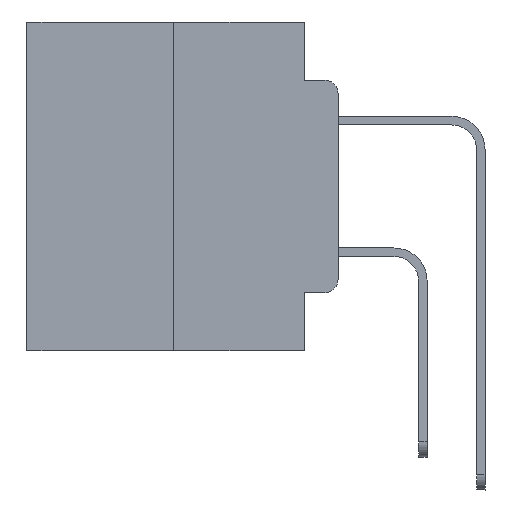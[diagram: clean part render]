
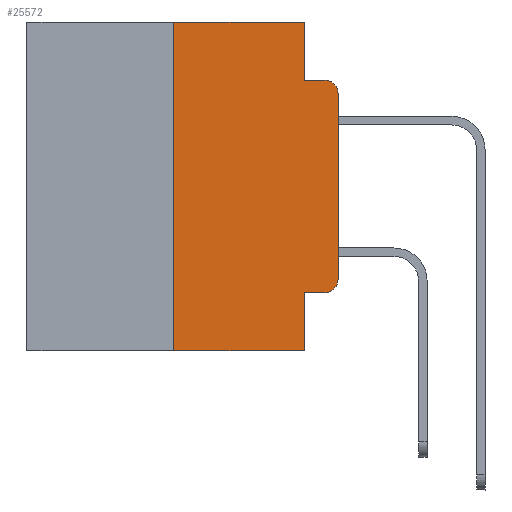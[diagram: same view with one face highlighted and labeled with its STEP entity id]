
A CAD part, left-side view. The second image highlights one B-rep face of the part: STEP entity #25572.
In plain terms, the highlighted planar face has unit normal (-1, 0, 0).
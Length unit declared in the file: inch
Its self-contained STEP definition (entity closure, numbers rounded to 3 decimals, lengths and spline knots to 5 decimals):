
#29 = DIRECTION ( 'NONE',  ( 0., -1., 0. ) ) ;
#83 = DIRECTION ( 'NONE',  ( 0., -1., 0. ) ) ;
#188 = EDGE_CURVE ( 'NONE', #13512, #18082, #9195, .T. ) ;
#240 = CARTESIAN_POINT ( 'NONE',  ( 0., 0.051, -0.0885 ) ) ;
#314 = CARTESIAN_POINT ( 'NONE',  ( 0., 0.02, -0.0885 ) ) ;
#466 = CARTESIAN_POINT ( 'NONE',  ( 0., 0.051, 0. ) ) ;
#577 = CARTESIAN_POINT ( 'NONE',  ( 0., 0.051, -0.0885 ) ) ;
#767 = CIRCLE ( 'NONE', #22059, 0.02 ) ;
#892 = CARTESIAN_POINT ( 'NONE',  ( 0., 0., 0. ) ) ;
#1604 = AXIS2_PLACEMENT_3D ( 'NONE', #3013, #21350, #19277 ) ;
#2238 = EDGE_CURVE ( 'NONE', #17097, #25896, #7556, .T. ) ;
#2462 = CARTESIAN_POINT ( 'NONE',  ( 0., 0.051, -0.4115 ) ) ;
#2566 = CARTESIAN_POINT ( 'NONE',  ( 0., 0.25, -0.5 ) ) ;
#3013 = CARTESIAN_POINT ( 'NONE',  ( 0., 0.02, -0.3915 ) ) ;
#3143 = CARTESIAN_POINT ( 'NONE',  ( 0., 0.25, 0. ) ) ;
#3380 = ORIENTED_EDGE ( 'NONE', *, *, #3652, .F. ) ;
#3582 = CARTESIAN_POINT ( 'NONE',  ( 0., 0.473, 0. ) ) ;
#3652 = EDGE_CURVE ( 'NONE', #5473, #27436, #4929, .T. ) ;
#3845 = CARTESIAN_POINT ( 'NONE',  ( 0., 0., -0.1085 ) ) ;
#3953 = VECTOR ( 'NONE', #27276, 39.37008 ) ;
#4034 = FACE_OUTER_BOUND ( 'NONE', #17146, .T. ) ;
#4355 = LINE ( 'NONE', #24919, #13659 ) ;
#4866 = CARTESIAN_POINT ( 'NONE',  ( 0., 0.25, 0. ) ) ;
#4929 = LINE ( 'NONE', #3143, #11040 ) ;
#5051 = ORIENTED_EDGE ( 'NONE', *, *, #12981, .T. ) ;
#5473 = VERTEX_POINT ( 'NONE', #2566 ) ;
#6499 = VERTEX_POINT ( 'NONE', #314 ) ;
#7221 = ORIENTED_EDGE ( 'NONE', *, *, #29108, .T. ) ;
#7556 = LINE ( 'NONE', #466, #18891 ) ;
#7664 = ORIENTED_EDGE ( 'NONE', *, *, #13264, .F. ) ;
#7984 = ORIENTED_EDGE ( 'NONE', *, *, #2238, .F. ) ;
#8680 = DIRECTION ( 'NONE',  ( -1., 0., 0. ) ) ;
#9007 = EDGE_CURVE ( 'NONE', #5473, #18082, #4355, .T. ) ;
#9189 = VERTEX_POINT ( 'NONE', #19699 ) ;
#9195 = LINE ( 'NONE', #18223, #3953 ) ;
#9214 = DIRECTION ( 'NONE',  ( 0., 0., 1. ) ) ;
#9650 = VERTEX_POINT ( 'NONE', #3845 ) ;
#10762 = CARTESIAN_POINT ( 'NONE',  ( 0., 0.02, -0.1085 ) ) ;
#10862 = DIRECTION ( 'NONE',  ( 0., -1., 0. ) ) ;
#11040 = VECTOR ( 'NONE', #9214, 39.37008 ) ;
#11886 = EDGE_CURVE ( 'NONE', #13512, #12898, #16207, .T. ) ;
#12185 = ORIENTED_EDGE ( 'NONE', *, *, #20729, .F. ) ;
#12315 = ORIENTED_EDGE ( 'NONE', *, *, #12469, .T. ) ;
#12469 = EDGE_CURVE ( 'NONE', #12898, #9189, #27140, .T. ) ;
#12898 = VERTEX_POINT ( 'NONE', #19241 ) ;
#12981 = EDGE_CURVE ( 'NONE', #9189, #9650, #23250, .T. ) ;
#13042 = PLANE ( 'NONE',  #25660 ) ;
#13235 = LINE ( 'NONE', #17503, #15631 ) ;
#13264 = EDGE_CURVE ( 'NONE', #25896, #6499, #22744, .T. ) ;
#13512 = VERTEX_POINT ( 'NONE', #26000 ) ;
#13659 = VECTOR ( 'NONE', #29, 39.37008 ) ;
#14627 = ORIENTED_EDGE ( 'NONE', *, *, #11886, .T. ) ;
#15631 = VECTOR ( 'NONE', #10862, 39.37008 ) ;
#15754 = CARTESIAN_POINT ( 'NONE',  ( 0., 0.051, -0.5 ) ) ;
#16207 = LINE ( 'NONE', #2462, #19534 ) ;
#17012 = DIRECTION ( 'NONE',  ( 0., 0., -1. ) ) ;
#17097 = VERTEX_POINT ( 'NONE', #19285 ) ;
#17146 = EDGE_LOOP ( 'NONE', ( #5051, #7221, #7664, #7984, #12185, #3380, #25011, #22921, #14627, #12315 ) ) ;
#17503 = CARTESIAN_POINT ( 'NONE',  ( 0., 0.473, 0. ) ) ;
#18082 = VERTEX_POINT ( 'NONE', #15754 ) ;
#18223 = CARTESIAN_POINT ( 'NONE',  ( 0., 0.051, 0. ) ) ;
#18236 = DIRECTION ( 'NONE',  ( 0., 0., -1. ) ) ;
#18891 = VECTOR ( 'NONE', #18236, 39.37008 ) ;
#19241 = CARTESIAN_POINT ( 'NONE',  ( 0., 0.02, -0.4115 ) ) ;
#19277 = DIRECTION ( 'NONE',  ( 0., 0., -1. ) ) ;
#19285 = CARTESIAN_POINT ( 'NONE',  ( 0., 0.051, 0. ) ) ;
#19534 = VECTOR ( 'NONE', #83, 39.37008 ) ;
#19699 = CARTESIAN_POINT ( 'NONE',  ( 0., 0., -0.3915 ) ) ;
#20729 = EDGE_CURVE ( 'NONE', #27436, #17097, #13235, .T. ) ;
#21350 = DIRECTION ( 'NONE',  ( -1., 0., 0. ) ) ;
#22059 = AXIS2_PLACEMENT_3D ( 'NONE', #10762, #8680, #28550 ) ;
#22559 = VECTOR ( 'NONE', #25273, 39.37008 ) ;
#22744 = LINE ( 'NONE', #240, #22559 ) ;
#22921 = ORIENTED_EDGE ( 'NONE', *, *, #188, .F. ) ;
#23250 = LINE ( 'NONE', #892, #28984 ) ;
#24919 = CARTESIAN_POINT ( 'NONE',  ( 0., 0.473, -0.5 ) ) ;
#25011 = ORIENTED_EDGE ( 'NONE', *, *, #9007, .T. ) ;
#25273 = DIRECTION ( 'NONE',  ( 0., -1., 0. ) ) ;
#25343 = DIRECTION ( 'NONE',  ( 0., 0., 1. ) ) ;
#25572 = ADVANCED_FACE ( 'NONE', ( #4034 ), #13042, .F. ) ;
#25660 = AXIS2_PLACEMENT_3D ( 'NONE', #3582, #28607, #17012 ) ;
#25896 = VERTEX_POINT ( 'NONE', #577 ) ;
#26000 = CARTESIAN_POINT ( 'NONE',  ( 0., 0.051, -0.4115 ) ) ;
#27140 = CIRCLE ( 'NONE', #1604, 0.02 ) ;
#27276 = DIRECTION ( 'NONE',  ( 0., 0., -1. ) ) ;
#27436 = VERTEX_POINT ( 'NONE', #4866 ) ;
#28550 = DIRECTION ( 'NONE',  ( 0., 0., -1. ) ) ;
#28607 = DIRECTION ( 'NONE',  ( 1., 0., 0. ) ) ;
#28984 = VECTOR ( 'NONE', #25343, 39.37008 ) ;
#29108 = EDGE_CURVE ( 'NONE', #9650, #6499, #767, .T. ) ;
